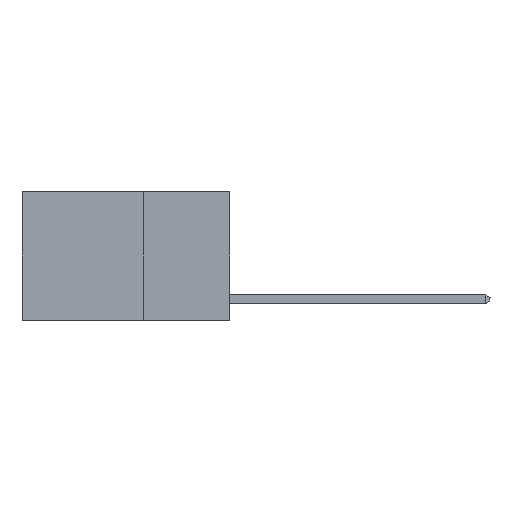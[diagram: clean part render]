
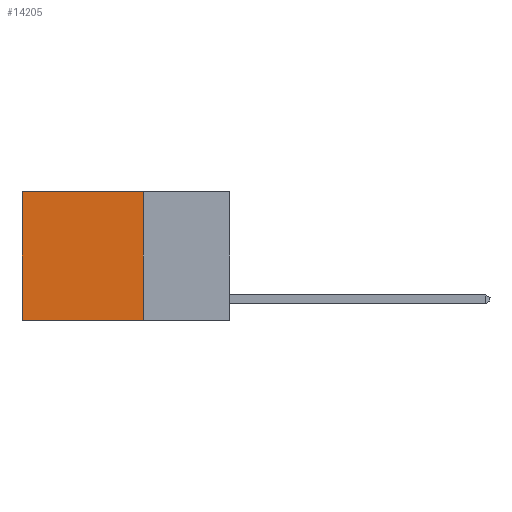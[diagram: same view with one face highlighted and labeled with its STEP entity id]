
A CAD part, left-side view. The second image highlights one B-rep face of the part: STEP entity #14205.
In plain terms, the highlighted planar face has unit normal (-1, 0, 0).
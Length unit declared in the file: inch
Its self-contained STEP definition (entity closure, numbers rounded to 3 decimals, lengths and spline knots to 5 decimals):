
#549 = CARTESIAN_POINT ( 'NONE',  ( 0.2625, 0.6, 0. ) ) ;
#1072 = AXIS2_PLACEMENT_3D ( 'NONE', #4345, #13038, #5594 ) ;
#1495 = CARTESIAN_POINT ( 'NONE',  ( 0.2625, 0.25, 0. ) ) ;
#1685 = CARTESIAN_POINT ( 'NONE',  ( 0.2625, 0.25, -0.37 ) ) ;
#1770 = EDGE_CURVE ( 'NONE', #9954, #6857, #8019, .T. ) ;
#1829 = ORIENTED_EDGE ( 'NONE', *, *, #11701, .T. ) ;
#1837 = PLANE ( 'NONE',  #1072 ) ;
#2393 = CARTESIAN_POINT ( 'NONE',  ( 0.2625, 0.25, 0. ) ) ;
#3062 = LINE ( 'NONE', #1495, #15834 ) ;
#3128 = EDGE_LOOP ( 'NONE', ( #7022, #3551, #5848, #1829 ) ) ;
#3551 = ORIENTED_EDGE ( 'NONE', *, *, #1770, .F. ) ;
#4328 = VECTOR ( 'NONE', #9138, 39.37008 ) ;
#4345 = CARTESIAN_POINT ( 'NONE',  ( 0.2625, 0.25, 0. ) ) ;
#4797 = VERTEX_POINT ( 'NONE', #2393 ) ;
#4987 = EDGE_CURVE ( 'NONE', #4797, #9954, #3062, .T. ) ;
#5188 = EDGE_CURVE ( 'NONE', #13628, #6857, #13157, .T. ) ;
#5447 = CARTESIAN_POINT ( 'NONE',  ( 0.2625, 0.25, 0. ) ) ;
#5594 = DIRECTION ( 'NONE',  ( 0., 0., -1. ) ) ;
#5848 = ORIENTED_EDGE ( 'NONE', *, *, #4987, .F. ) ;
#6541 = VECTOR ( 'NONE', #15437, 39.37008 ) ;
#6857 = VERTEX_POINT ( 'NONE', #11302 ) ;
#7022 = ORIENTED_EDGE ( 'NONE', *, *, #5188, .T. ) ;
#7131 = CARTESIAN_POINT ( 'NONE',  ( 0.2625, 0.25, -0.37 ) ) ;
#7998 = LINE ( 'NONE', #5447, #14200 ) ;
#8019 = LINE ( 'NONE', #1685, #4328 ) ;
#8949 = DIRECTION ( 'NONE',  ( 0., 0., -1. ) ) ;
#9138 = DIRECTION ( 'NONE',  ( 0., 1., 0. ) ) ;
#9954 = VERTEX_POINT ( 'NONE', #7131 ) ;
#10727 = FACE_OUTER_BOUND ( 'NONE', #3128, .T. ) ;
#11302 = CARTESIAN_POINT ( 'NONE',  ( 0.2625, 0.6, -0.37 ) ) ;
#11659 = DIRECTION ( 'NONE',  ( 0., 1., 0. ) ) ;
#11701 = EDGE_CURVE ( 'NONE', #4797, #13628, #7998, .T. ) ;
#13038 = DIRECTION ( 'NONE',  ( 1., 0., 0. ) ) ;
#13157 = LINE ( 'NONE', #549, #6541 ) ;
#13628 = VERTEX_POINT ( 'NONE', #14337 ) ;
#14200 = VECTOR ( 'NONE', #11659, 39.37008 ) ;
#14205 = ADVANCED_FACE ( 'NONE', ( #10727 ), #1837, .F. ) ;
#14337 = CARTESIAN_POINT ( 'NONE',  ( 0.2625, 0.6, 0. ) ) ;
#15437 = DIRECTION ( 'NONE',  ( 0., 0., -1. ) ) ;
#15834 = VECTOR ( 'NONE', #8949, 39.37008 ) ;
